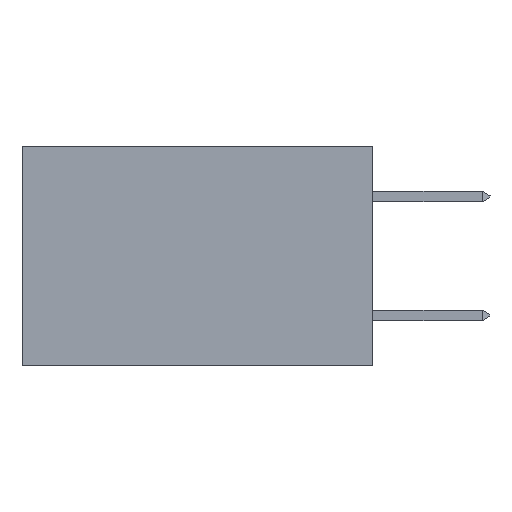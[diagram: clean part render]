
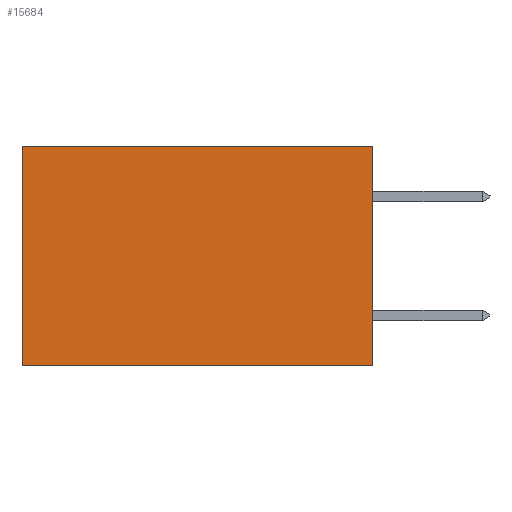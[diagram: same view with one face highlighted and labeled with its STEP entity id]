
A CAD part, left-side view. The second image highlights one B-rep face of the part: STEP entity #15684.
In plain terms, the highlighted planar face has unit normal (-1, 0, 0).
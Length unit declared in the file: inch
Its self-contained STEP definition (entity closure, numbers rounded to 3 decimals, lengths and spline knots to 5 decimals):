
#2992 = ORIENTED_EDGE ( 'NONE', *, *, #21390, .F. ) ;
#3002 = CARTESIAN_POINT ( 'NONE',  ( 0.277, 0., 0. ) ) ;
#3366 = ORIENTED_EDGE ( 'NONE', *, *, #7678, .F. ) ;
#3393 = AXIS2_PLACEMENT_3D ( 'NONE', #17279, #30589, #14694 ) ;
#4000 = PLANE ( 'NONE',  #3393 ) ;
#6529 = LINE ( 'NONE', #29529, #26864 ) ;
#7678 = EDGE_CURVE ( 'NONE', #16709, #19486, #27842, .T. ) ;
#7872 = DIRECTION ( 'NONE',  ( 0., 1., 0. ) ) ;
#8948 = DIRECTION ( 'NONE',  ( 0., 0., -1. ) ) ;
#9147 = EDGE_LOOP ( 'NONE', ( #18606, #2992, #3366, #9266 ) ) ;
#9266 = ORIENTED_EDGE ( 'NONE', *, *, #26375, .T. ) ;
#10546 = VECTOR ( 'NONE', #8948, 39.37008 ) ;
#10674 = CARTESIAN_POINT ( 'NONE',  ( 0.277, 0.59, -0.37 ) ) ;
#14247 = CARTESIAN_POINT ( 'NONE',  ( 0.277, 0., -0.37 ) ) ;
#14694 = DIRECTION ( 'NONE',  ( 0., 0., -1. ) ) ;
#15684 = ADVANCED_FACE ( 'NONE', ( #34278 ), #4000, .F. ) ;
#15742 = CARTESIAN_POINT ( 'NONE',  ( 0.277, 0., -0.37 ) ) ;
#16709 = VERTEX_POINT ( 'NONE', #3002 ) ;
#16813 = CARTESIAN_POINT ( 'NONE',  ( 0.277, 0.59, -0.37 ) ) ;
#17279 = CARTESIAN_POINT ( 'NONE',  ( 0.277, 0., -0.37 ) ) ;
#18386 = VECTOR ( 'NONE', #7872, 39.37008 ) ;
#18606 = ORIENTED_EDGE ( 'NONE', *, *, #20979, .T. ) ;
#19486 = VERTEX_POINT ( 'NONE', #14247 ) ;
#20979 = EDGE_CURVE ( 'NONE', #29289, #23762, #24640, .T. ) ;
#21390 = EDGE_CURVE ( 'NONE', #19486, #23762, #26286, .T. ) ;
#21619 = VECTOR ( 'NONE', #30024, 39.37008 ) ;
#22067 = CARTESIAN_POINT ( 'NONE',  ( 0.277, 0., -0.37 ) ) ;
#22448 = CARTESIAN_POINT ( 'NONE',  ( 0.277, 0.59, 0. ) ) ;
#23762 = VERTEX_POINT ( 'NONE', #10674 ) ;
#24640 = LINE ( 'NONE', #16813, #10546 ) ;
#26286 = LINE ( 'NONE', #15742, #18386 ) ;
#26375 = EDGE_CURVE ( 'NONE', #16709, #29289, #6529, .T. ) ;
#26864 = VECTOR ( 'NONE', #26870, 39.37008 ) ;
#26870 = DIRECTION ( 'NONE',  ( 0., 1., 0. ) ) ;
#27842 = LINE ( 'NONE', #22067, #21619 ) ;
#29289 = VERTEX_POINT ( 'NONE', #22448 ) ;
#29529 = CARTESIAN_POINT ( 'NONE',  ( 0.277, 0., 0. ) ) ;
#30024 = DIRECTION ( 'NONE',  ( 0., 0., -1. ) ) ;
#30589 = DIRECTION ( 'NONE',  ( 1., 0., 0. ) ) ;
#34278 = FACE_OUTER_BOUND ( 'NONE', #9147, .T. ) ;
